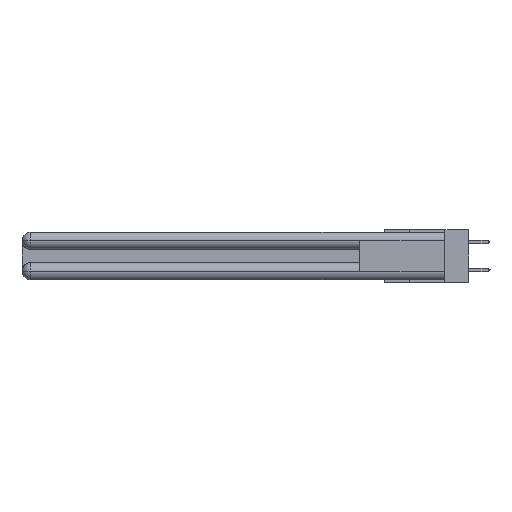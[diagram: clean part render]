
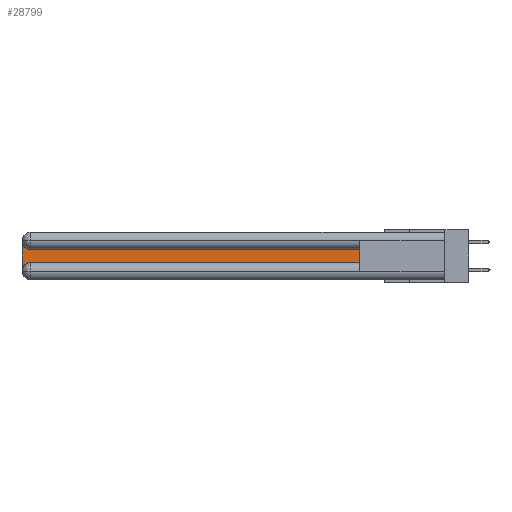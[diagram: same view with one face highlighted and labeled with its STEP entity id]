
A CAD part, left-side view. The second image highlights one B-rep face of the part: STEP entity #28799.
In plain terms, the highlighted planar face has unit normal (-1, 0, 0).
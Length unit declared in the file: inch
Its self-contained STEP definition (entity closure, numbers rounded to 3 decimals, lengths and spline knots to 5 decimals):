
#647 = VECTOR ( 'NONE', #21242, 39.37008 ) ;
#1335 = VERTEX_POINT ( 'NONE', #11022 ) ;
#2498 = CARTESIAN_POINT ( 'NONE',  ( 0.075, 3., -0.0625 ) ) ;
#2745 = EDGE_CURVE ( 'NONE', #13207, #1335, #22335, .T. ) ;
#4102 = CARTESIAN_POINT ( 'NONE',  ( 0.075, 3., -0.2175 ) ) ;
#4802 = ORIENTED_EDGE ( 'NONE', *, *, #25970, .T. ) ;
#4983 = VERTEX_POINT ( 'NONE', #20496 ) ;
#5039 = DIRECTION ( 'NONE',  ( 0., 1., 0. ) ) ;
#5241 = DIRECTION ( 'NONE',  ( 1., 0., 0. ) ) ;
#5859 = AXIS2_PLACEMENT_3D ( 'NONE', #21418, #6802, #26321 ) ;
#6802 = DIRECTION ( 'NONE',  ( 1., 0., 0. ) ) ;
#6993 = EDGE_CURVE ( 'NONE', #28951, #23080, #22434, .T. ) ;
#7059 = AXIS2_PLACEMENT_3D ( 'NONE', #12590, #5241, #29628 ) ;
#7684 = CARTESIAN_POINT ( 'NONE',  ( 0.075, 0.6, -0.1225 ) ) ;
#7783 = DIRECTION ( 'NONE',  ( 0., -1., 0. ) ) ;
#10130 = VECTOR ( 'NONE', #27908, 39.37008 ) ;
#11022 = CARTESIAN_POINT ( 'NONE',  ( 0.075, 0.6, -0.1225 ) ) ;
#12144 = FACE_OUTER_BOUND ( 'NONE', #24718, .T. ) ;
#12590 = CARTESIAN_POINT ( 'NONE',  ( 0.075, 3., -0.1225 ) ) ;
#13207 = VERTEX_POINT ( 'NONE', #31405 ) ;
#14590 = DIRECTION ( 'NONE',  ( 0., 0., -1. ) ) ;
#14743 = AXIS2_PLACEMENT_3D ( 'NONE', #31347, #26672, #14590 ) ;
#14989 = ORIENTED_EDGE ( 'NONE', *, *, #19243, .T. ) ;
#15120 = PLANE ( 'NONE',  #7059 ) ;
#15834 = EDGE_CURVE ( 'NONE', #4983, #16367, #23050, .T. ) ;
#15911 = VECTOR ( 'NONE', #7783, 39.37008 ) ;
#16367 = VERTEX_POINT ( 'NONE', #28325 ) ;
#18462 = VECTOR ( 'NONE', #5039, 39.37008 ) ;
#19243 = EDGE_CURVE ( 'NONE', #16367, #13207, #20102, .T. ) ;
#19949 = CARTESIAN_POINT ( 'NONE',  ( 0.075, 0.6, -0.2175 ) ) ;
#20102 = LINE ( 'NONE', #19949, #15911 ) ;
#20340 = CARTESIAN_POINT ( 'NONE',  ( 0.075, 0.6, -0.2175 ) ) ;
#20496 = CARTESIAN_POINT ( 'NONE',  ( 0.075, 3., -0.2775 ) ) ;
#20580 = ORIENTED_EDGE ( 'NONE', *, *, #2745, .T. ) ;
#21242 = DIRECTION ( 'NONE',  ( 0., 0., -1. ) ) ;
#21418 = CARTESIAN_POINT ( 'NONE',  ( 0.075, 2.94, -0.0625 ) ) ;
#22309 = CARTESIAN_POINT ( 'NONE',  ( 0.075, 2.94, -0.1225 ) ) ;
#22335 = LINE ( 'NONE', #20340, #10130 ) ;
#22434 = CIRCLE ( 'NONE', #5859, 0.06 ) ;
#22860 = ORIENTED_EDGE ( 'NONE', *, *, #26237, .T. ) ;
#23050 = CIRCLE ( 'NONE', #14743, 0.06 ) ;
#23080 = VERTEX_POINT ( 'NONE', #2498 ) ;
#24718 = EDGE_LOOP ( 'NONE', ( #22860, #28893, #4802, #27545, #14989, #20580 ) ) ;
#24990 = LINE ( 'NONE', #4102, #647 ) ;
#25970 = EDGE_CURVE ( 'NONE', #23080, #4983, #24990, .T. ) ;
#26237 = EDGE_CURVE ( 'NONE', #1335, #28951, #30284, .T. ) ;
#26321 = DIRECTION ( 'NONE',  ( 0., 0., -1. ) ) ;
#26672 = DIRECTION ( 'NONE',  ( 1., 0., 0. ) ) ;
#27545 = ORIENTED_EDGE ( 'NONE', *, *, #15834, .T. ) ;
#27908 = DIRECTION ( 'NONE',  ( 0., 0., 1. ) ) ;
#28325 = CARTESIAN_POINT ( 'NONE',  ( 0.075, 2.94, -0.2175 ) ) ;
#28799 = ADVANCED_FACE ( 'NONE', ( #12144 ), #15120, .F. ) ;
#28893 = ORIENTED_EDGE ( 'NONE', *, *, #6993, .T. ) ;
#28951 = VERTEX_POINT ( 'NONE', #22309 ) ;
#29628 = DIRECTION ( 'NONE',  ( 0., 0., -1. ) ) ;
#30284 = LINE ( 'NONE', #7684, #18462 ) ;
#31347 = CARTESIAN_POINT ( 'NONE',  ( 0.075, 2.94, -0.2775 ) ) ;
#31405 = CARTESIAN_POINT ( 'NONE',  ( 0.075, 0.6, -0.2175 ) ) ;
